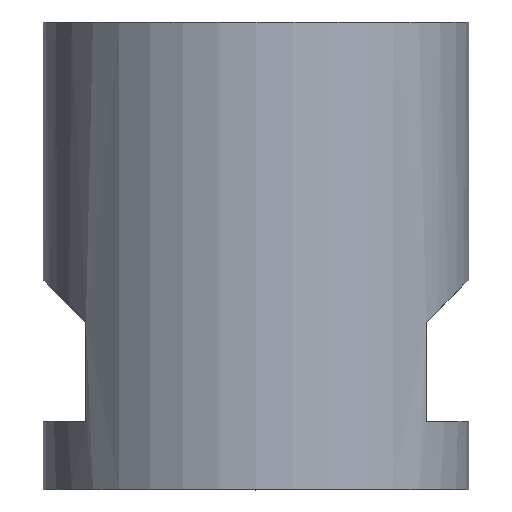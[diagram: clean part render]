
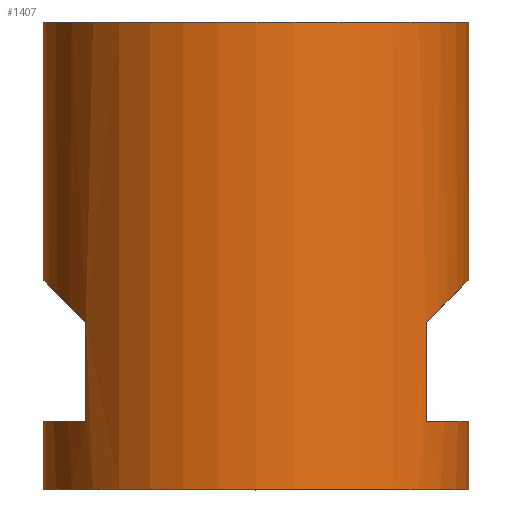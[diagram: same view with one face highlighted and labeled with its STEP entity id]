
A CAD part, top view. The second image highlights one B-rep face of the part: STEP entity #1407.
In plain terms, the highlighted cylindrical face has radius 18.123 mm (diameter 36.246 mm), a full revolution.
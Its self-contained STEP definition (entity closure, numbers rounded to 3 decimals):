
#67=FACE_BOUND('',#261,.T.);
#68=ELLIPSE('',#1429,25.63,18.123);
#69=ELLIPSE('',#1430,25.63,18.123);
#70=ELLIPSE('',#1433,25.63,18.123);
#71=ELLIPSE('',#1434,25.63,18.123);
#176=FACE_OUTER_BOUND('',#260,.T.);
#260=EDGE_LOOP('',(#1293,#1294,#1295,#1296,#1297,#1298,#1299,#1300,#1301,
#1302,#1303,#1304,#1305,#1306));
#261=EDGE_LOOP('',(#1307,#1308,#1309,#1310,#1311,#1312));
#264=CIRCLE('',#1437,18.123);
#265=CIRCLE('',#1439,18.123);
#266=CIRCLE('',#1440,18.123);
#267=CIRCLE('',#1442,18.123);
#268=CIRCLE('',#1443,18.123);
#272=CIRCLE('',#1449,18.123);
#296=CIRCLE('',#1539,18.123);
#297=CIRCLE('',#1541,18.123);
#387=LINE('',#2352,#471);
#389=LINE('',#2355,#473);
#392=LINE('',#2367,#476);
#394=LINE('',#2370,#478);
#462=LINE('',#3618,#546);
#463=LINE('',#3619,#547);
#471=VECTOR('',#1570,10.);
#473=VECTOR('',#1572,10.);
#476=VECTOR('',#1583,10.);
#478=VECTOR('',#1585,10.);
#546=VECTOR('',#1863,18.123);
#547=VECTOR('',#1864,18.123);
#576=VERTEX_POINT('',#2342);
#577=VERTEX_POINT('',#2343);
#578=VERTEX_POINT('',#2345);
#579=VERTEX_POINT('',#2347);
#580=VERTEX_POINT('',#2351);
#581=VERTEX_POINT('',#2353);
#582=VERTEX_POINT('',#2357);
#583=VERTEX_POINT('',#2358);
#584=VERTEX_POINT('',#2360);
#585=VERTEX_POINT('',#2362);
#586=VERTEX_POINT('',#2366);
#587=VERTEX_POINT('',#2368);
#588=VERTEX_POINT('',#2374);
#589=VERTEX_POINT('',#2378);
#593=VERTEX_POINT('',#2390);
#681=VERTEX_POINT('',#3615);
#712=EDGE_CURVE('',#576,#577,#68,.T.);
#714=EDGE_CURVE('',#578,#579,#69,.T.);
#716=EDGE_CURVE('',#580,#577,#387,.T.);
#718=EDGE_CURVE('',#578,#581,#389,.T.);
#719=EDGE_CURVE('',#582,#583,#70,.T.);
#721=EDGE_CURVE('',#584,#585,#71,.T.);
#723=EDGE_CURVE('',#586,#585,#392,.T.);
#725=EDGE_CURVE('',#583,#587,#394,.T.);
#726=EDGE_CURVE('',#584,#582,#264,.T.);
#727=EDGE_CURVE('',#588,#579,#265,.T.);
#728=EDGE_CURVE('',#576,#588,#266,.T.);
#729=EDGE_CURVE('',#589,#580,#267,.T.);
#730=EDGE_CURVE('',#581,#589,#268,.T.);
#735=EDGE_CURVE('',#593,#593,#272,.T.);
#889=EDGE_CURVE('',#681,#681,#296,.T.);
#890=EDGE_CURVE('',#593,#588,#462,.T.);
#891=EDGE_CURVE('',#589,#681,#463,.T.);
#892=EDGE_CURVE('',#587,#586,#297,.T.);
#1293=ORIENTED_EDGE('',*,*,#735,.F.);
#1294=ORIENTED_EDGE('',*,*,#890,.T.);
#1295=ORIENTED_EDGE('',*,*,#727,.T.);
#1296=ORIENTED_EDGE('',*,*,#714,.F.);
#1297=ORIENTED_EDGE('',*,*,#718,.T.);
#1298=ORIENTED_EDGE('',*,*,#730,.T.);
#1299=ORIENTED_EDGE('',*,*,#891,.T.);
#1300=ORIENTED_EDGE('',*,*,#889,.F.);
#1301=ORIENTED_EDGE('',*,*,#891,.F.);
#1302=ORIENTED_EDGE('',*,*,#729,.T.);
#1303=ORIENTED_EDGE('',*,*,#716,.T.);
#1304=ORIENTED_EDGE('',*,*,#712,.F.);
#1305=ORIENTED_EDGE('',*,*,#728,.T.);
#1306=ORIENTED_EDGE('',*,*,#890,.F.);
#1307=ORIENTED_EDGE('',*,*,#721,.F.);
#1308=ORIENTED_EDGE('',*,*,#726,.T.);
#1309=ORIENTED_EDGE('',*,*,#719,.T.);
#1310=ORIENTED_EDGE('',*,*,#725,.T.);
#1311=ORIENTED_EDGE('',*,*,#892,.T.);
#1312=ORIENTED_EDGE('',*,*,#723,.T.);
#1327=CYLINDRICAL_SURFACE('',#1540,18.123);
#1407=ADVANCED_FACE('',(#176,#67),#1327,.T.);
#1429=AXIS2_PLACEMENT_3D('',#2344,#1562,#1563);
#1430=AXIS2_PLACEMENT_3D('',#2348,#1565,#1566);
#1433=AXIS2_PLACEMENT_3D('',#2359,#1575,#1576);
#1434=AXIS2_PLACEMENT_3D('',#2363,#1578,#1579);
#1437=AXIS2_PLACEMENT_3D('',#2372,#1588,#1589);
#1439=AXIS2_PLACEMENT_3D('',#2375,#1592,#1593);
#1440=AXIS2_PLACEMENT_3D('',#2376,#1594,#1595);
#1442=AXIS2_PLACEMENT_3D('',#2379,#1598,#1599);
#1443=AXIS2_PLACEMENT_3D('',#2380,#1600,#1601);
#1449=AXIS2_PLACEMENT_3D('',#2391,#1613,#1614);
#1539=AXIS2_PLACEMENT_3D('',#3616,#1859,#1860);
#1540=AXIS2_PLACEMENT_3D('',#3617,#1861,#1862);
#1541=AXIS2_PLACEMENT_3D('',#3620,#1865,#1866);
#1562=DIRECTION('center_axis',(-0.707,-0.707,0.));
#1563=DIRECTION('ref_axis',(0.707,-0.707,0.));
#1565=DIRECTION('center_axis',(-0.707,-0.707,0.));
#1566=DIRECTION('ref_axis',(0.707,-0.707,0.));
#1570=DIRECTION('',(0.,1.,0.));
#1572=DIRECTION('',(0.,-1.,0.));
#1575=DIRECTION('center_axis',(-0.707,0.707,0.));
#1576=DIRECTION('ref_axis',(0.707,0.707,0.));
#1578=DIRECTION('center_axis',(0.707,-0.707,0.));
#1579=DIRECTION('ref_axis',(0.707,0.707,0.));
#1583=DIRECTION('',(0.,1.,0.));
#1585=DIRECTION('',(0.,-1.,0.));
#1588=DIRECTION('center_axis',(0.,1.,0.));
#1589=DIRECTION('ref_axis',(1.,0.,0.));
#1592=DIRECTION('center_axis',(0.,1.,0.));
#1593=DIRECTION('ref_axis',(1.,0.,0.));
#1594=DIRECTION('center_axis',(0.,1.,0.));
#1595=DIRECTION('ref_axis',(1.,0.,0.));
#1598=DIRECTION('center_axis',(0.,-1.,0.));
#1599=DIRECTION('ref_axis',(1.,0.,0.));
#1600=DIRECTION('center_axis',(0.,-1.,0.));
#1601=DIRECTION('ref_axis',(1.,0.,0.));
#1613=DIRECTION('center_axis',(0.,1.,0.));
#1614=DIRECTION('ref_axis',(1.,0.,0.));
#1859=DIRECTION('center_axis',(0.,-1.,0.));
#1860=DIRECTION('ref_axis',(1.,0.,0.));
#1861=DIRECTION('center_axis',(0.,1.,0.));
#1862=DIRECTION('ref_axis',(1.,0.,0.));
#1863=DIRECTION('',(0.,-1.,0.));
#1864=DIRECTION('',(0.,-1.,0.));
#1865=DIRECTION('center_axis',(0.,-1.,0.));
#1866=DIRECTION('ref_axis',(1.,0.,0.));
#2342=CARTESIAN_POINT('',(-18.044,-153.057,-33.347));
#2343=CARTESIAN_POINT('',(-14.488,-156.613,-42.455));
#2344=CARTESIAN_POINT('Origin',(-0.01,-171.091,
-31.554));
#2345=CARTESIAN_POINT('',(-14.488,-156.613,-20.654));
#2347=CARTESIAN_POINT('',(-18.044,-153.057,-29.761));
#2348=CARTESIAN_POINT('Origin',(-0.01,-171.091,
-31.554));
#2351=CARTESIAN_POINT('',(-14.488,-165.021,-42.455));
#2352=CARTESIAN_POINT('',(-14.488,-170.827,-42.455));
#2353=CARTESIAN_POINT('',(-14.488,-165.021,-20.654));
#2355=CARTESIAN_POINT('',(-14.488,-170.827,-20.654));
#2357=CARTESIAN_POINT('',(18.024,-153.057,-33.347));
#2358=CARTESIAN_POINT('',(14.468,-156.613,-42.455));
#2359=CARTESIAN_POINT('Origin',(-0.01,-171.091,
-31.554));
#2360=CARTESIAN_POINT('',(18.024,-153.057,-29.761));
#2362=CARTESIAN_POINT('',(14.468,-156.613,-20.654));
#2363=CARTESIAN_POINT('Origin',(-0.01,-171.091,
-31.554));
#2366=CARTESIAN_POINT('',(14.468,-165.021,-20.654));
#2367=CARTESIAN_POINT('',(14.468,-170.827,-20.654));
#2368=CARTESIAN_POINT('',(14.468,-165.021,-42.455));
#2370=CARTESIAN_POINT('',(14.468,-170.827,-42.455));
#2372=CARTESIAN_POINT('Origin',(-0.01,-153.057,
-31.554));
#2374=CARTESIAN_POINT('',(-18.132,-153.057,-31.554));
#2375=CARTESIAN_POINT('Origin',(-0.01,-153.057,
-31.554));
#2376=CARTESIAN_POINT('Origin',(-0.01,-153.057,
-31.554));
#2378=CARTESIAN_POINT('',(-18.132,-165.021,-31.554));
#2379=CARTESIAN_POINT('Origin',(-0.01,-165.021,
-31.554));
#2380=CARTESIAN_POINT('Origin',(-0.01,-165.021,
-31.554));
#2390=CARTESIAN_POINT('',(-18.132,-131.05,-31.554));
#2391=CARTESIAN_POINT('Origin',(-0.01,-131.05,-31.554));
#3615=CARTESIAN_POINT('',(-18.132,-170.827,-31.554));
#3616=CARTESIAN_POINT('Origin',(-0.01,-170.827,
-31.554));
#3617=CARTESIAN_POINT('Origin',(-0.01,-170.827,
-31.554));
#3618=CARTESIAN_POINT('',(-18.132,-170.827,-31.554));
#3619=CARTESIAN_POINT('',(-18.132,-170.827,-31.554));
#3620=CARTESIAN_POINT('Origin',(-0.01,-165.021,
-31.554));
